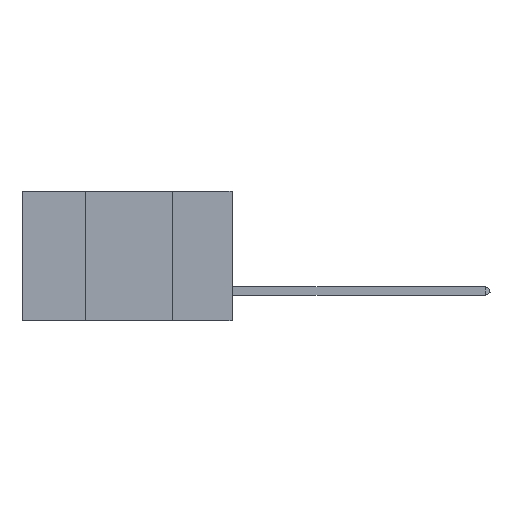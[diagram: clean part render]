
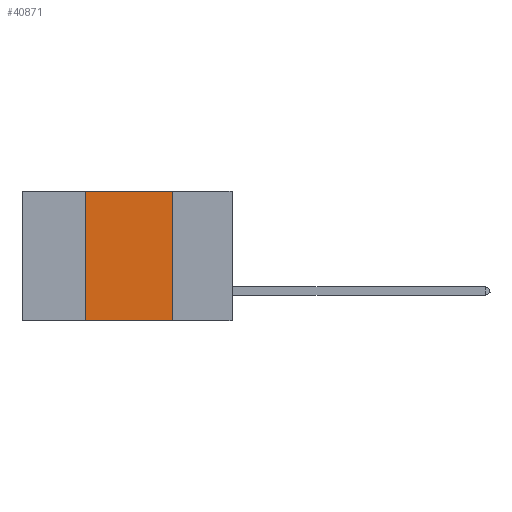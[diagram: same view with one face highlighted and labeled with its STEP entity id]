
A CAD part, left-side view. The second image highlights one B-rep face of the part: STEP entity #40871.
In plain terms, the highlighted planar face has unit normal (-1, 0, 0).
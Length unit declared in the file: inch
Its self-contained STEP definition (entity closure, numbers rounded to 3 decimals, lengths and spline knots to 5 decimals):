
#1211 = ORIENTED_EDGE ( 'NONE', *, *, #15078, .F. ) ;
#4202 = DIRECTION ( 'NONE',  ( 0., -1., 0. ) ) ;
#4393 = CARTESIAN_POINT ( 'NONE',  ( 0., 0.6, 0. ) ) ;
#7495 = LINE ( 'NONE', #12243, #42573 ) ;
#8143 = PLANE ( 'NONE',  #22616 ) ;
#8375 = VERTEX_POINT ( 'NONE', #19413 ) ;
#9975 = EDGE_LOOP ( 'NONE', ( #12997, #10100, #1211, #26292 ) ) ;
#10100 = ORIENTED_EDGE ( 'NONE', *, *, #22068, .F. ) ;
#10852 = DIRECTION ( 'NONE',  ( 0., 0., -1. ) ) ;
#11369 = DIRECTION ( 'NONE',  ( 1., 0., 0. ) ) ;
#12243 = CARTESIAN_POINT ( 'NONE',  ( 0., 0.42, 0. ) ) ;
#12997 = ORIENTED_EDGE ( 'NONE', *, *, #43648, .F. ) ;
#13147 = FACE_OUTER_BOUND ( 'NONE', #9975, .T. ) ;
#13674 = LINE ( 'NONE', #31948, #37816 ) ;
#15078 = EDGE_CURVE ( 'NONE', #26400, #23568, #7495, .T. ) ;
#15387 = VECTOR ( 'NONE', #10852, 39.37008 ) ;
#18698 = LINE ( 'NONE', #27716, #15387 ) ;
#19413 = CARTESIAN_POINT ( 'NONE',  ( 0., 0.17, -0.37 ) ) ;
#21773 = VECTOR ( 'NONE', #4202, 39.37008 ) ;
#22068 = EDGE_CURVE ( 'NONE', #23568, #33437, #28348, .T. ) ;
#22616 = AXIS2_PLACEMENT_3D ( 'NONE', #4393, #11369, #36149 ) ;
#23568 = VERTEX_POINT ( 'NONE', #36030 ) ;
#26292 = ORIENTED_EDGE ( 'NONE', *, *, #44313, .T. ) ;
#26400 = VERTEX_POINT ( 'NONE', #39659 ) ;
#27716 = CARTESIAN_POINT ( 'NONE',  ( 0., 0.17, 0. ) ) ;
#28348 = LINE ( 'NONE', #42884, #21773 ) ;
#31948 = CARTESIAN_POINT ( 'NONE',  ( 0., 0.6, -0.37 ) ) ;
#33437 = VERTEX_POINT ( 'NONE', #33841 ) ;
#33841 = CARTESIAN_POINT ( 'NONE',  ( 0., 0.17, 0. ) ) ;
#36030 = CARTESIAN_POINT ( 'NONE',  ( 0., 0.42, 0. ) ) ;
#36149 = DIRECTION ( 'NONE',  ( 0., 0., -1. ) ) ;
#37816 = VECTOR ( 'NONE', #42205, 39.37008 ) ;
#37965 = DIRECTION ( 'NONE',  ( 0., 0., 1. ) ) ;
#39659 = CARTESIAN_POINT ( 'NONE',  ( 0., 0.42, -0.37 ) ) ;
#40871 = ADVANCED_FACE ( 'NONE', ( #13147 ), #8143, .F. ) ;
#42205 = DIRECTION ( 'NONE',  ( 0., -1., 0. ) ) ;
#42573 = VECTOR ( 'NONE', #37965, 39.37008 ) ;
#42884 = CARTESIAN_POINT ( 'NONE',  ( 0., 0.6, 0. ) ) ;
#43648 = EDGE_CURVE ( 'NONE', #33437, #8375, #18698, .T. ) ;
#44313 = EDGE_CURVE ( 'NONE', #26400, #8375, #13674, .T. ) ;
